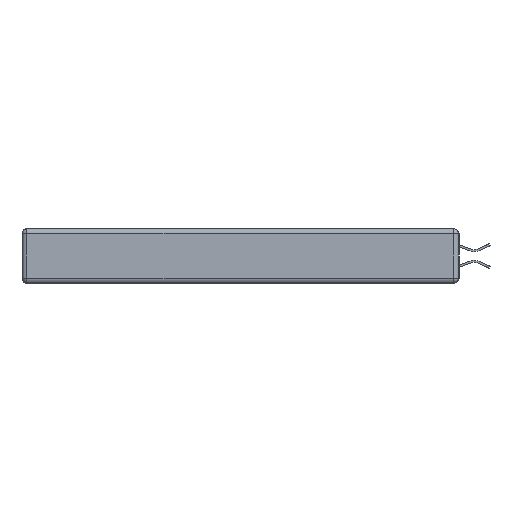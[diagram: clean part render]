
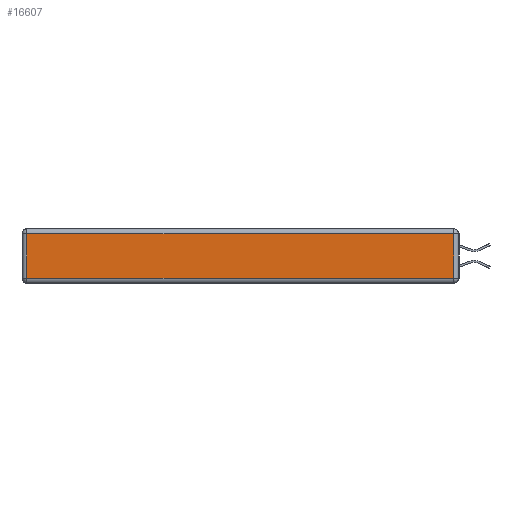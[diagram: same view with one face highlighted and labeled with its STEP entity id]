
A CAD part, left-side view. The second image highlights one B-rep face of the part: STEP entity #16607.
In plain terms, the highlighted planar face has unit normal (-1, 0, 0).
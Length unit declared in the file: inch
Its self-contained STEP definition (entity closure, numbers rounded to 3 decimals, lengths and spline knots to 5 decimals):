
#46 = VECTOR ( 'NONE', #24609, 39.37008 ) ;
#583 = CARTESIAN_POINT ( 'NONE',  ( 0., 0., -0.343 ) ) ;
#736 = EDGE_CURVE ( 'NONE', #15417, #11095, #9713, .T. ) ;
#1502 = CARTESIAN_POINT ( 'NONE',  ( 0., 0.03, -0.313 ) ) ;
#1773 = VERTEX_POINT ( 'NONE', #1502 ) ;
#1974 = DIRECTION ( 'NONE',  ( 0., -1., 0. ) ) ;
#2910 = ORIENTED_EDGE ( 'NONE', *, *, #8983, .T. ) ;
#3021 = FACE_OUTER_BOUND ( 'NONE', #11244, .T. ) ;
#5778 = CARTESIAN_POINT ( 'NONE',  ( 0., 0.03, -0.03 ) ) ;
#5985 = CARTESIAN_POINT ( 'NONE',  ( 0., 0., -0.313 ) ) ;
#6449 = VERTEX_POINT ( 'NONE', #5778 ) ;
#7229 = LINE ( 'NONE', #21334, #18961 ) ;
#8983 = EDGE_CURVE ( 'NONE', #11095, #1773, #20929, .T. ) ;
#9713 = LINE ( 'NONE', #17432, #17968 ) ;
#11095 = VERTEX_POINT ( 'NONE', #20120 ) ;
#11244 = EDGE_LOOP ( 'NONE', ( #2910, #25166, #25730, #19156 ) ) ;
#11574 = DIRECTION ( 'NONE',  ( 0., 0., 1. ) ) ;
#11922 = CARTESIAN_POINT ( 'NONE',  ( 0., 2.72, -0.03 ) ) ;
#12455 = DIRECTION ( 'NONE',  ( 0., 0., 1. ) ) ;
#15417 = VERTEX_POINT ( 'NONE', #11922 ) ;
#16238 = LINE ( 'NONE', #25670, #46 ) ;
#16607 = ADVANCED_FACE ( 'NONE', ( #3021 ), #22986, .T. ) ;
#17432 = CARTESIAN_POINT ( 'NONE',  ( 0., 2.72, -0.343 ) ) ;
#17968 = VECTOR ( 'NONE', #25661, 39.37008 ) ;
#18961 = VECTOR ( 'NONE', #11574, 39.37008 ) ;
#19156 = ORIENTED_EDGE ( 'NONE', *, *, #736, .T. ) ;
#20120 = CARTESIAN_POINT ( 'NONE',  ( 0., 2.72, -0.313 ) ) ;
#20397 = AXIS2_PLACEMENT_3D ( 'NONE', #583, #20818, #12455 ) ;
#20818 = DIRECTION ( 'NONE',  ( -1., 0., 0. ) ) ;
#20929 = LINE ( 'NONE', #5985, #21917 ) ;
#21334 = CARTESIAN_POINT ( 'NONE',  ( 0., 0.03, -0.343 ) ) ;
#21467 = EDGE_CURVE ( 'NONE', #6449, #15417, #16238, .T. ) ;
#21917 = VECTOR ( 'NONE', #1974, 39.37008 ) ;
#22986 = PLANE ( 'NONE',  #20397 ) ;
#24609 = DIRECTION ( 'NONE',  ( 0., 1., 0. ) ) ;
#25166 = ORIENTED_EDGE ( 'NONE', *, *, #26344, .T. ) ;
#25661 = DIRECTION ( 'NONE',  ( 0., 0., -1. ) ) ;
#25670 = CARTESIAN_POINT ( 'NONE',  ( 0., 2.75, -0.03 ) ) ;
#25730 = ORIENTED_EDGE ( 'NONE', *, *, #21467, .T. ) ;
#26344 = EDGE_CURVE ( 'NONE', #1773, #6449, #7229, .T. ) ;
